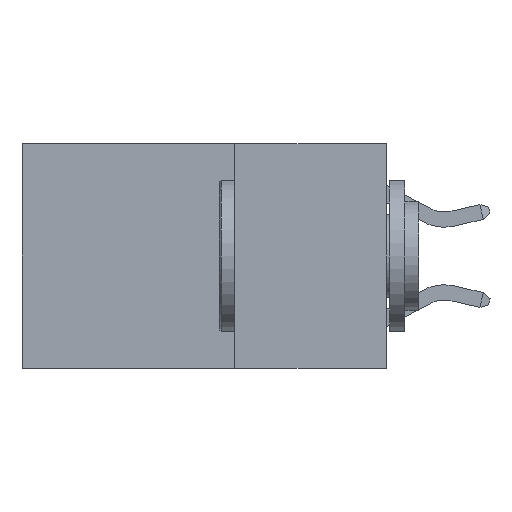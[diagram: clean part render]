
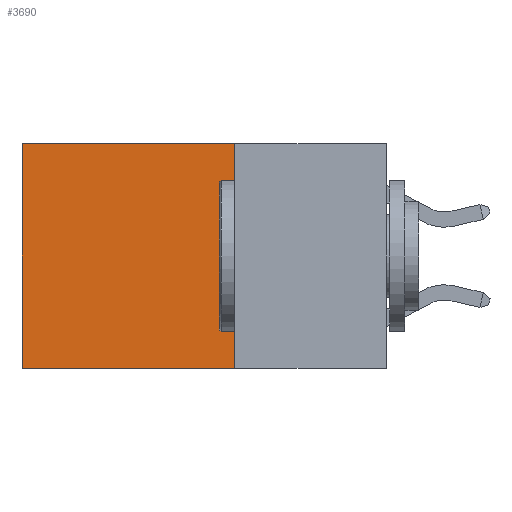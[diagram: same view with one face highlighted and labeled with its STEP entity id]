
A CAD part, left-side view. The second image highlights one B-rep face of the part: STEP entity #3690.
In plain terms, the highlighted planar face has unit normal (-1, 0, 0).
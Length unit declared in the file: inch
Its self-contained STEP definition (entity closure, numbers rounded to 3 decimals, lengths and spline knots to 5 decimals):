
#142 = DIRECTION ( 'NONE',  ( 0., 0., -1. ) ) ;
#2586 = VERTEX_POINT ( 'NONE', #12244 ) ;
#2917 = LINE ( 'NONE', #11441, #8179 ) ;
#3690 = ADVANCED_FACE ( 'NONE', ( #8778 ), #13232, .F. ) ;
#4126 = LINE ( 'NONE', #9779, #13298 ) ;
#4240 = CARTESIAN_POINT ( 'NONE',  ( 0.2625, 0.25, -0.37 ) ) ;
#4403 = VECTOR ( 'NONE', #12692, 39.37008 ) ;
#4604 = CARTESIAN_POINT ( 'NONE',  ( 0.2625, 0.25, 0. ) ) ;
#5126 = EDGE_LOOP ( 'NONE', ( #8647, #15224, #16358, #14876 ) ) ;
#5443 = LINE ( 'NONE', #4240, #4403 ) ;
#8179 = VECTOR ( 'NONE', #11260, 39.37008 ) ;
#8647 = ORIENTED_EDGE ( 'NONE', *, *, #9640, .T. ) ;
#8778 = FACE_OUTER_BOUND ( 'NONE', #5126, .T. ) ;
#8949 = DIRECTION ( 'NONE',  ( 1., 0., 0. ) ) ;
#9640 = EDGE_CURVE ( 'NONE', #10119, #11150, #10168, .T. ) ;
#9779 = CARTESIAN_POINT ( 'NONE',  ( 0.2625, 0.25, 0. ) ) ;
#9878 = CARTESIAN_POINT ( 'NONE',  ( 0.2625, 0.6, 0. ) ) ;
#10119 = VERTEX_POINT ( 'NONE', #9878 ) ;
#10168 = LINE ( 'NONE', #12961, #16134 ) ;
#10586 = CARTESIAN_POINT ( 'NONE',  ( 0.2625, 0.25, 0. ) ) ;
#10647 = VERTEX_POINT ( 'NONE', #10586 ) ;
#11150 = VERTEX_POINT ( 'NONE', #13257 ) ;
#11260 = DIRECTION ( 'NONE',  ( 0., 1., 0. ) ) ;
#11441 = CARTESIAN_POINT ( 'NONE',  ( 0.2625, 0.25, 0. ) ) ;
#11563 = DIRECTION ( 'NONE',  ( 0., 0., -1. ) ) ;
#12244 = CARTESIAN_POINT ( 'NONE',  ( 0.2625, 0.25, -0.37 ) ) ;
#12692 = DIRECTION ( 'NONE',  ( 0., 1., 0. ) ) ;
#12758 = DIRECTION ( 'NONE',  ( 0., 0., -1. ) ) ;
#12961 = CARTESIAN_POINT ( 'NONE',  ( 0.2625, 0.6, 0. ) ) ;
#13025 = AXIS2_PLACEMENT_3D ( 'NONE', #4604, #8949, #142 ) ;
#13232 = PLANE ( 'NONE',  #13025 ) ;
#13257 = CARTESIAN_POINT ( 'NONE',  ( 0.2625, 0.6, -0.37 ) ) ;
#13298 = VECTOR ( 'NONE', #12758, 39.37008 ) ;
#13410 = EDGE_CURVE ( 'NONE', #10647, #10119, #2917, .T. ) ;
#14876 = ORIENTED_EDGE ( 'NONE', *, *, #13410, .T. ) ;
#15224 = ORIENTED_EDGE ( 'NONE', *, *, #17813, .F. ) ;
#16134 = VECTOR ( 'NONE', #11563, 39.37008 ) ;
#16358 = ORIENTED_EDGE ( 'NONE', *, *, #18320, .F. ) ;
#17813 = EDGE_CURVE ( 'NONE', #2586, #11150, #5443, .T. ) ;
#18320 = EDGE_CURVE ( 'NONE', #10647, #2586, #4126, .T. ) ;
